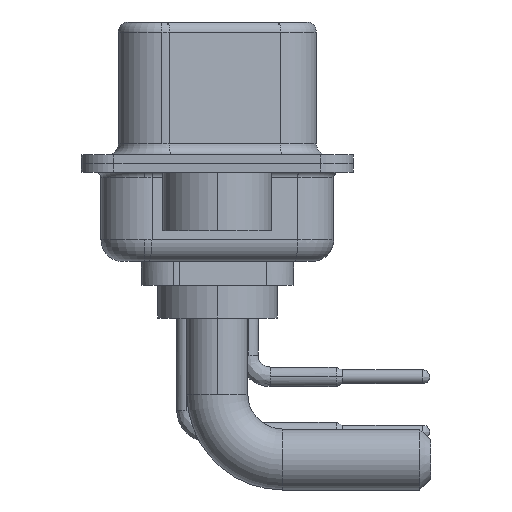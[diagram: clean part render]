
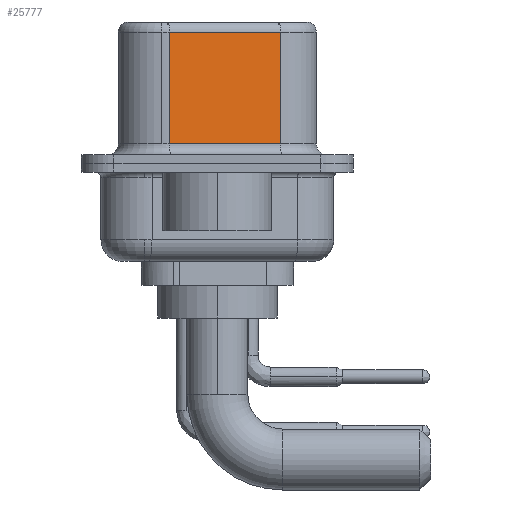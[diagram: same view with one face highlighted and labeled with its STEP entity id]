
A CAD part, left-side view. The second image highlights one B-rep face of the part: STEP entity #25777.
In plain terms, the highlighted planar face has unit normal (-0.985, -0.174, 0).
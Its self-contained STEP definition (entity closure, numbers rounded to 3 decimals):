
#576 = ORIENTED_EDGE ( 'NONE', *, *, #10855, .F. ) ;
#649 = DIRECTION ( 'NONE',  ( 0., 0., -1. ) ) ;
#1637 = CARTESIAN_POINT ( 'NONE',  ( 4.58, -2.897, 6.02 ) ) ;
#2334 = CARTESIAN_POINT ( 'NONE',  ( 3.68, 2.203, 6.02 ) ) ;
#3227 = LINE ( 'NONE', #22903, #18999 ) ;
#6269 = DIRECTION ( 'NONE',  ( 0.985, 0.174, 0. ) ) ;
#6588 = VECTOR ( 'NONE', #649, 1000. ) ;
#7581 = LINE ( 'NONE', #26817, #6588 ) ;
#8246 = DIRECTION ( 'NONE',  ( 0., 0., -1. ) ) ;
#8579 = LINE ( 'NONE', #1637, #22660 ) ;
#9386 = EDGE_LOOP ( 'NONE', ( #576, #28302, #18815, #9655 ) ) ;
#9655 = ORIENTED_EDGE ( 'NONE', *, *, #11648, .T. ) ;
#10565 = LINE ( 'NONE', #19237, #15745 ) ;
#10855 = EDGE_CURVE ( 'NONE', #11428, #17323, #10565, .T. ) ;
#11176 = CARTESIAN_POINT ( 'NONE',  ( 4.58, -2.897, 0.9 ) ) ;
#11428 = VERTEX_POINT ( 'NONE', #14295 ) ;
#11648 = EDGE_CURVE ( 'NONE', #14486, #17323, #3227, .T. ) ;
#13973 = EDGE_CURVE ( 'NONE', #18322, #14486, #7581, .T. ) ;
#14295 = CARTESIAN_POINT ( 'NONE',  ( 4.58, -2.897, 6.02 ) ) ;
#14486 = VERTEX_POINT ( 'NONE', #20702 ) ;
#14952 = CARTESIAN_POINT ( 'NONE',  ( 4.58, -2.897, 6.52 ) ) ;
#15745 = VECTOR ( 'NONE', #8246, 1000. ) ;
#16825 = DIRECTION ( 'NONE',  ( -0.174, 0.985, 0. ) ) ;
#17264 = PLANE ( 'NONE',  #20859 ) ;
#17323 = VERTEX_POINT ( 'NONE', #11176 ) ;
#18322 = VERTEX_POINT ( 'NONE', #2334 ) ;
#18815 = ORIENTED_EDGE ( 'NONE', *, *, #13973, .T. ) ;
#18999 = VECTOR ( 'NONE', #25361, 1000. ) ;
#19237 = CARTESIAN_POINT ( 'NONE',  ( 4.58, -2.897, 6.52 ) ) ;
#20702 = CARTESIAN_POINT ( 'NONE',  ( 3.68, 2.203, 0.9 ) ) ;
#20859 = AXIS2_PLACEMENT_3D ( 'NONE', #14952, #6269, #23779 ) ;
#22660 = VECTOR ( 'NONE', #16825, 1000. ) ;
#22903 = CARTESIAN_POINT ( 'NONE',  ( 4.58, -2.897, 0.9 ) ) ;
#23284 = EDGE_CURVE ( 'NONE', #11428, #18322, #8579, .T. ) ;
#23639 = FACE_OUTER_BOUND ( 'NONE', #9386, .T. ) ;
#23779 = DIRECTION ( 'NONE',  ( -0.174, 0.985, 0. ) ) ;
#25361 = DIRECTION ( 'NONE',  ( 0.174, -0.985, 0. ) ) ;
#25777 = ADVANCED_FACE ( 'NONE', ( #23639 ), #17264, .F. ) ;
#26817 = CARTESIAN_POINT ( 'NONE',  ( 3.68, 2.203, 6.52 ) ) ;
#28302 = ORIENTED_EDGE ( 'NONE', *, *, #23284, .T. ) ;
